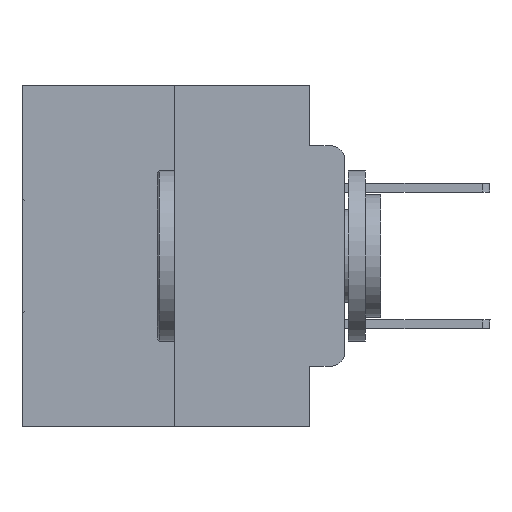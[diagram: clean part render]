
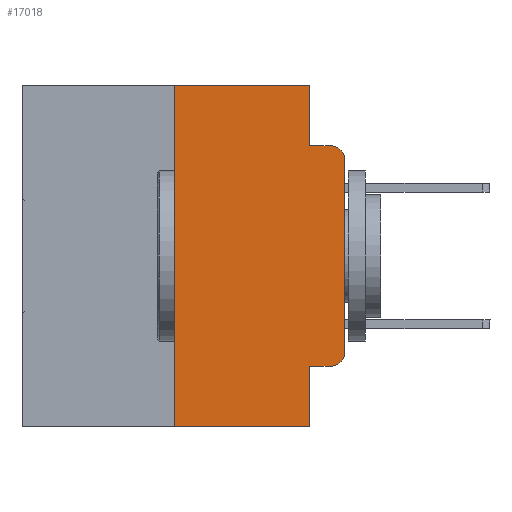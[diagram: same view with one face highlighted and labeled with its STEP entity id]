
A CAD part, left-side view. The second image highlights one B-rep face of the part: STEP entity #17018.
In plain terms, the highlighted planar face has unit normal (-1, 0, 0).
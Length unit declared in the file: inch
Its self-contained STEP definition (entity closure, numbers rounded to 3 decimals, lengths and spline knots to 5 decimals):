
#287 = ORIENTED_EDGE ( 'NONE', *, *, #6833, .T. ) ;
#1212 = VECTOR ( 'NONE', #29452, 39.37008 ) ;
#1218 = CARTESIAN_POINT ( 'NONE',  ( 0., 0., -0.3915 ) ) ;
#1367 = CARTESIAN_POINT ( 'NONE',  ( 0., 0.473, 0. ) ) ;
#1666 = ORIENTED_EDGE ( 'NONE', *, *, #9266, .T. ) ;
#1908 = LINE ( 'NONE', #8419, #28722 ) ;
#2260 = VECTOR ( 'NONE', #5050, 39.37008 ) ;
#2583 = LINE ( 'NONE', #12054, #2260 ) ;
#2831 = CARTESIAN_POINT ( 'NONE',  ( 0., 0.051, -0.5 ) ) ;
#3559 = CARTESIAN_POINT ( 'NONE',  ( 0., 0.02, -0.3915 ) ) ;
#4200 = CARTESIAN_POINT ( 'NONE',  ( 0., 0.051, 0. ) ) ;
#4621 = CARTESIAN_POINT ( 'NONE',  ( 0., 0.051, 0. ) ) ;
#5003 = CARTESIAN_POINT ( 'NONE',  ( 0., 0., 0. ) ) ;
#5050 = DIRECTION ( 'NONE',  ( 0., -1., 0. ) ) ;
#6170 = ORIENTED_EDGE ( 'NONE', *, *, #12237, .T. ) ;
#6188 = DIRECTION ( 'NONE',  ( -1., 0., 0. ) ) ;
#6233 = AXIS2_PLACEMENT_3D ( 'NONE', #1367, #25166, #18005 ) ;
#6833 = EDGE_CURVE ( 'NONE', #30031, #11402, #24357, .T. ) ;
#7264 = CARTESIAN_POINT ( 'NONE',  ( 0., 0.02, -0.4115 ) ) ;
#8341 = ORIENTED_EDGE ( 'NONE', *, *, #22316, .F. ) ;
#8419 = CARTESIAN_POINT ( 'NONE',  ( 0., 0.473, 0. ) ) ;
#8558 = EDGE_CURVE ( 'NONE', #30031, #12194, #10445, .T. ) ;
#9266 = EDGE_CURVE ( 'NONE', #18052, #29706, #2583, .T. ) ;
#9591 = ORIENTED_EDGE ( 'NONE', *, *, #13842, .T. ) ;
#10445 = LINE ( 'NONE', #19946, #1212 ) ;
#10528 = VERTEX_POINT ( 'NONE', #1218 ) ;
#10746 = CARTESIAN_POINT ( 'NONE',  ( 0., 0.051, -0.0885 ) ) ;
#10843 = CARTESIAN_POINT ( 'NONE',  ( 0., 0.051, 0. ) ) ;
#11153 = LINE ( 'NONE', #23468, #26197 ) ;
#11402 = VERTEX_POINT ( 'NONE', #2831 ) ;
#11707 = EDGE_CURVE ( 'NONE', #18052, #11402, #25515, .T. ) ;
#12054 = CARTESIAN_POINT ( 'NONE',  ( 0., 0.051, -0.4115 ) ) ;
#12194 = VERTEX_POINT ( 'NONE', #28575 ) ;
#12237 = EDGE_CURVE ( 'NONE', #18304, #13583, #14240, .T. ) ;
#12706 = EDGE_CURVE ( 'NONE', #14037, #13583, #11153, .T. ) ;
#13158 = FACE_OUTER_BOUND ( 'NONE', #21684, .T. ) ;
#13171 = DIRECTION ( 'NONE',  ( 0., 0., -1. ) ) ;
#13583 = VERTEX_POINT ( 'NONE', #20129 ) ;
#13788 = ORIENTED_EDGE ( 'NONE', *, *, #24448, .F. ) ;
#13806 = DIRECTION ( 'NONE',  ( 0., -1., 0. ) ) ;
#13842 = EDGE_CURVE ( 'NONE', #10528, #18304, #28664, .T. ) ;
#14037 = VERTEX_POINT ( 'NONE', #10746 ) ;
#14217 = ORIENTED_EDGE ( 'NONE', *, *, #29359, .T. ) ;
#14240 = CIRCLE ( 'NONE', #29664, 0.02 ) ;
#14268 = DIRECTION ( 'NONE',  ( -1., 0., 0. ) ) ;
#14413 = CARTESIAN_POINT ( 'NONE',  ( 0., 0.02, -0.1085 ) ) ;
#14495 = AXIS2_PLACEMENT_3D ( 'NONE', #3559, #6188, #22695 ) ;
#14709 = DIRECTION ( 'NONE',  ( 0., -1., 0. ) ) ;
#14818 = VECTOR ( 'NONE', #14709, 39.37008 ) ;
#16989 = CIRCLE ( 'NONE', #14495, 0.02 ) ;
#17018 = ADVANCED_FACE ( 'NONE', ( #13158 ), #22676, .F. ) ;
#17079 = VECTOR ( 'NONE', #28055, 39.37008 ) ;
#17708 = ORIENTED_EDGE ( 'NONE', *, *, #11707, .F. ) ;
#17923 = DIRECTION ( 'NONE',  ( 0., -1., 0. ) ) ;
#18005 = DIRECTION ( 'NONE',  ( 0., 0., -1. ) ) ;
#18052 = VERTEX_POINT ( 'NONE', #28031 ) ;
#18217 = CARTESIAN_POINT ( 'NONE',  ( 0., 0., -0.1085 ) ) ;
#18304 = VERTEX_POINT ( 'NONE', #18217 ) ;
#18497 = ORIENTED_EDGE ( 'NONE', *, *, #12706, .F. ) ;
#19233 = CARTESIAN_POINT ( 'NONE',  ( 0., 0.473, -0.5 ) ) ;
#19946 = CARTESIAN_POINT ( 'NONE',  ( 0., 0.25, 0. ) ) ;
#20129 = CARTESIAN_POINT ( 'NONE',  ( 0., 0.02, -0.0885 ) ) ;
#20501 = ORIENTED_EDGE ( 'NONE', *, *, #8558, .F. ) ;
#21425 = DIRECTION ( 'NONE',  ( 0., 0., -1. ) ) ;
#21684 = EDGE_LOOP ( 'NONE', ( #9591, #6170, #18497, #13788, #8341, #20501, #287, #17708, #1666, #14217 ) ) ;
#22316 = EDGE_CURVE ( 'NONE', #12194, #29583, #1908, .T. ) ;
#22676 = PLANE ( 'NONE',  #6233 ) ;
#22695 = DIRECTION ( 'NONE',  ( 0., 0., -1. ) ) ;
#23196 = DIRECTION ( 'NONE',  ( 0., 0., -1. ) ) ;
#23468 = CARTESIAN_POINT ( 'NONE',  ( 0., 0.051, -0.0885 ) ) ;
#24357 = LINE ( 'NONE', #19233, #14818 ) ;
#24448 = EDGE_CURVE ( 'NONE', #29583, #14037, #25328, .T. ) ;
#25166 = DIRECTION ( 'NONE',  ( 1., 0., 0. ) ) ;
#25308 = VECTOR ( 'NONE', #13171, 39.37008 ) ;
#25328 = LINE ( 'NONE', #10843, #25308 ) ;
#25515 = LINE ( 'NONE', #4200, #26705 ) ;
#26197 = VECTOR ( 'NONE', #13806, 39.37008 ) ;
#26705 = VECTOR ( 'NONE', #23196, 39.37008 ) ;
#27935 = CARTESIAN_POINT ( 'NONE',  ( 0., 0.25, -0.5 ) ) ;
#28031 = CARTESIAN_POINT ( 'NONE',  ( 0., 0.051, -0.4115 ) ) ;
#28055 = DIRECTION ( 'NONE',  ( 0., 0., 1. ) ) ;
#28575 = CARTESIAN_POINT ( 'NONE',  ( 0., 0.25, 0. ) ) ;
#28664 = LINE ( 'NONE', #5003, #17079 ) ;
#28722 = VECTOR ( 'NONE', #17923, 39.37008 ) ;
#29359 = EDGE_CURVE ( 'NONE', #29706, #10528, #16989, .T. ) ;
#29452 = DIRECTION ( 'NONE',  ( 0., 0., 1. ) ) ;
#29583 = VERTEX_POINT ( 'NONE', #4621 ) ;
#29664 = AXIS2_PLACEMENT_3D ( 'NONE', #14413, #14268, #21425 ) ;
#29706 = VERTEX_POINT ( 'NONE', #7264 ) ;
#30031 = VERTEX_POINT ( 'NONE', #27935 ) ;
